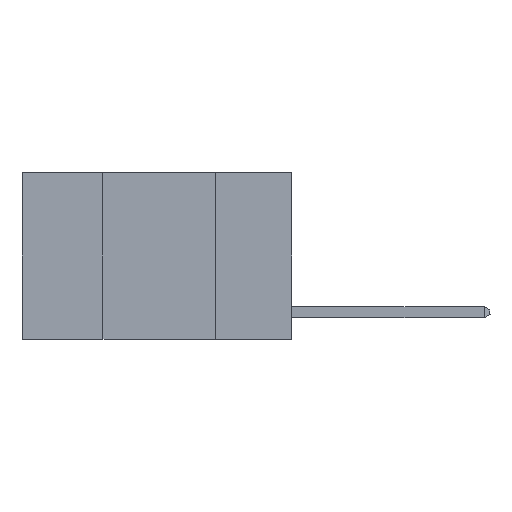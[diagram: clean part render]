
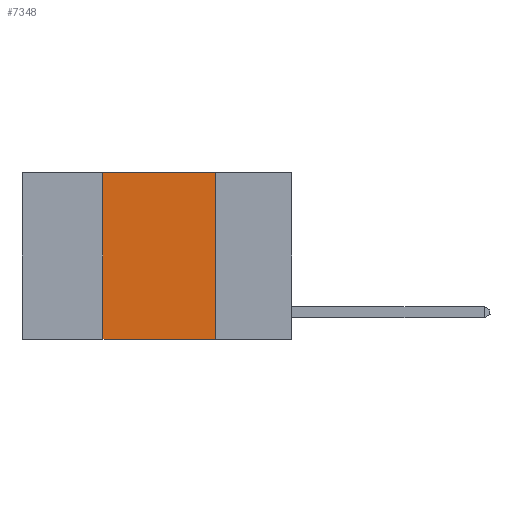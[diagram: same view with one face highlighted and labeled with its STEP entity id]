
A CAD part, left-side view. The second image highlights one B-rep face of the part: STEP entity #7348.
In plain terms, the highlighted planar face has unit normal (-1, 0, 0).
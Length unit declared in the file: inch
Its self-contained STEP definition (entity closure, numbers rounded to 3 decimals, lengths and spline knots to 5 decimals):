
#157 = LINE ( 'NONE', #2202, #3167 ) ;
#168 = VECTOR ( 'NONE', #4818, 39.37008 ) ;
#343 = DIRECTION ( 'NONE',  ( 0., -1., 0. ) ) ;
#431 = FACE_OUTER_BOUND ( 'NONE', #5606, .T. ) ;
#478 = CARTESIAN_POINT ( 'NONE',  ( 0., 0.17, -0.37 ) ) ;
#905 = CARTESIAN_POINT ( 'NONE',  ( 0., 0.6, 0. ) ) ;
#1544 = CARTESIAN_POINT ( 'NONE',  ( 0., 0.17, 0. ) ) ;
#1646 = AXIS2_PLACEMENT_3D ( 'NONE', #5226, #1904, #7215 ) ;
#1904 = DIRECTION ( 'NONE',  ( 1., 0., 0. ) ) ;
#2012 = VERTEX_POINT ( 'NONE', #8241 ) ;
#2179 = VERTEX_POINT ( 'NONE', #478 ) ;
#2202 = CARTESIAN_POINT ( 'NONE',  ( 0., 0.42, 0. ) ) ;
#2631 = CARTESIAN_POINT ( 'NONE',  ( 0., 0.42, -0.37 ) ) ;
#2986 = DIRECTION ( 'NONE',  ( 0., 0., 1. ) ) ;
#3125 = VERTEX_POINT ( 'NONE', #2631 ) ;
#3167 = VECTOR ( 'NONE', #2986, 39.37008 ) ;
#3284 = CARTESIAN_POINT ( 'NONE',  ( 0., 0.6, -0.37 ) ) ;
#4041 = ORIENTED_EDGE ( 'NONE', *, *, #4076, .F. ) ;
#4066 = DIRECTION ( 'NONE',  ( 0., -1., 0. ) ) ;
#4076 = EDGE_CURVE ( 'NONE', #2012, #2179, #7421, .T. ) ;
#4309 = LINE ( 'NONE', #905, #4576 ) ;
#4576 = VECTOR ( 'NONE', #343, 39.37008 ) ;
#4645 = LINE ( 'NONE', #3284, #4680 ) ;
#4680 = VECTOR ( 'NONE', #4066, 39.37008 ) ;
#4796 = ORIENTED_EDGE ( 'NONE', *, *, #6401, .F. ) ;
#4818 = DIRECTION ( 'NONE',  ( 0., 0., -1. ) ) ;
#5226 = CARTESIAN_POINT ( 'NONE',  ( 0., 0.6, 0. ) ) ;
#5461 = VERTEX_POINT ( 'NONE', #6539 ) ;
#5592 = EDGE_CURVE ( 'NONE', #3125, #2179, #4645, .T. ) ;
#5606 = EDGE_LOOP ( 'NONE', ( #4041, #7131, #4796, #7378 ) ) ;
#6401 = EDGE_CURVE ( 'NONE', #3125, #5461, #157, .T. ) ;
#6539 = CARTESIAN_POINT ( 'NONE',  ( 0., 0.42, 0. ) ) ;
#7131 = ORIENTED_EDGE ( 'NONE', *, *, #7332, .F. ) ;
#7215 = DIRECTION ( 'NONE',  ( 0., 0., -1. ) ) ;
#7332 = EDGE_CURVE ( 'NONE', #5461, #2012, #4309, .T. ) ;
#7348 = ADVANCED_FACE ( 'NONE', ( #431 ), #7891, .F. ) ;
#7378 = ORIENTED_EDGE ( 'NONE', *, *, #5592, .T. ) ;
#7421 = LINE ( 'NONE', #1544, #168 ) ;
#7891 = PLANE ( 'NONE',  #1646 ) ;
#8241 = CARTESIAN_POINT ( 'NONE',  ( 0., 0.17, 0. ) ) ;
